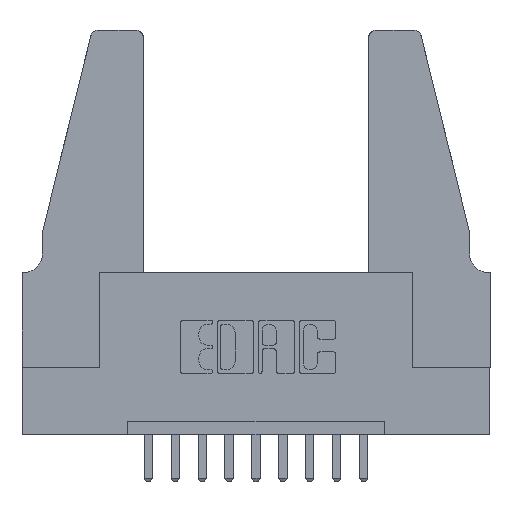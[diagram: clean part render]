
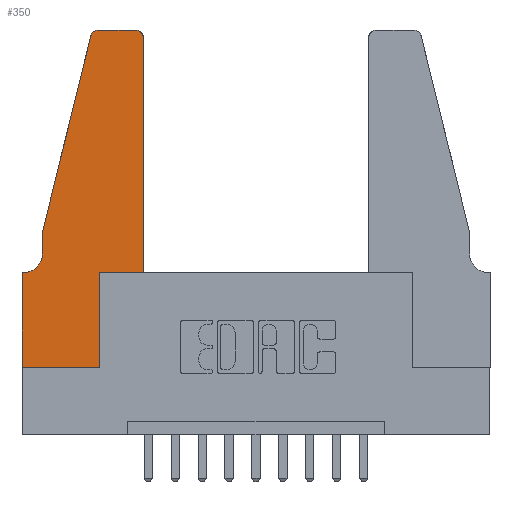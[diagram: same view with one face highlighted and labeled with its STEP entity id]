
A CAD part, top view. The second image highlights one B-rep face of the part: STEP entity #350.
In plain terms, the highlighted planar face has unit normal (0, 0, 1).
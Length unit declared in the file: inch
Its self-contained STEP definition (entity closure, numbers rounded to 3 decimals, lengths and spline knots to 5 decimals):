
#40 = EDGE_CURVE ( 'NONE', #12148, #10804, #7948, .T. ) ;
#112 = CARTESIAN_POINT ( 'NONE',  ( 0.2865, 0., 0.37 ) ) ;
#146 = DIRECTION ( 'NONE',  ( 0., 0., 1. ) ) ;
#165 = DIRECTION ( 'NONE',  ( 0., 0., 1. ) ) ;
#336 = LINE ( 'NONE', #9665, #4794 ) ;
#350 = ADVANCED_FACE ( 'NONE', ( #13003 ), #9407, .T. ) ;
#484 = VERTEX_POINT ( 'NONE', #9982 ) ;
#587 = CARTESIAN_POINT ( 'NONE',  ( 0.4505, 0.35, 0.37 ) ) ;
#904 = ORIENTED_EDGE ( 'NONE', *, *, #8625, .T. ) ;
#1178 = EDGE_CURVE ( 'NONE', #2941, #2637, #1564, .T. ) ;
#1369 = ORIENTED_EDGE ( 'NONE', *, *, #12515, .T. ) ;
#1439 = CARTESIAN_POINT ( 'NONE',  ( 0.0755, 0.5, 0.37 ) ) ;
#1564 = LINE ( 'NONE', #9667, #9541 ) ;
#1947 = CARTESIAN_POINT ( 'NONE',  ( 0.0755, 0.5, 0.37 ) ) ;
#2086 = LINE ( 'NONE', #9489, #12978 ) ;
#2240 = CARTESIAN_POINT ( 'NONE',  ( 0.0055, 0.42, 0.37 ) ) ;
#2256 = LINE ( 'NONE', #587, #9693 ) ;
#2637 = VERTEX_POINT ( 'NONE', #3068 ) ;
#2775 = DIRECTION ( 'NONE',  ( 1., 0., 0. ) ) ;
#2941 = VERTEX_POINT ( 'NONE', #12126 ) ;
#3068 = CARTESIAN_POINT ( 'NONE',  ( 0.4505, 1.22, 0.37 ) ) ;
#3259 = CARTESIAN_POINT ( 'NONE',  ( 0.0055, 0.35, 0.37 ) ) ;
#3442 = DIRECTION ( 'NONE',  ( -1., 0., 0. ) ) ;
#3523 = AXIS2_PLACEMENT_3D ( 'NONE', #9601, #165, #10624 ) ;
#3945 = ORIENTED_EDGE ( 'NONE', *, *, #1178, .T. ) ;
#4208 = CARTESIAN_POINT ( 'NONE',  ( 0.2605, 1.25, 0.37 ) ) ;
#4266 = VECTOR ( 'NONE', #6578, 39.37008 ) ;
#4300 = CARTESIAN_POINT ( 'NONE',  ( 0.284, 1.25, 0.37 ) ) ;
#4306 = EDGE_CURVE ( 'NONE', #10760, #12148, #11775, .T. ) ;
#4363 = VERTEX_POINT ( 'NONE', #8695 ) ;
#4393 = DIRECTION ( 'NONE',  ( 0., 0., -1. ) ) ;
#4583 = VECTOR ( 'NONE', #5790, 39.37008 ) ;
#4794 = VECTOR ( 'NONE', #3442, 39.37008 ) ;
#5053 = ORIENTED_EDGE ( 'NONE', *, *, #9400, .T. ) ;
#5328 = VERTEX_POINT ( 'NONE', #3259 ) ;
#5356 = VERTEX_POINT ( 'NONE', #4300 ) ;
#5540 = LINE ( 'NONE', #4208, #12079 ) ;
#5725 = CIRCLE ( 'NONE', #3523, 0.03 ) ;
#5748 = CARTESIAN_POINT ( 'NONE',  ( 0.2865, 0.35, 0.37 ) ) ;
#5778 = DIRECTION ( 'NONE',  ( 0., 0., 1. ) ) ;
#5790 = DIRECTION ( 'NONE',  ( 0., 1., 0. ) ) ;
#5828 = DIRECTION ( 'NONE',  ( 1., 0., 0. ) ) ;
#6429 = DIRECTION ( 'NONE',  ( 0., 1., 0. ) ) ;
#6578 = DIRECTION ( 'NONE',  ( -0.239, -0.971, 0. ) ) ;
#6589 = EDGE_CURVE ( 'NONE', #5328, #4363, #336, .T. ) ;
#6986 = ORIENTED_EDGE ( 'NONE', *, *, #8814, .T. ) ;
#7058 = EDGE_CURVE ( 'NONE', #13311, #10262, #9336, .T. ) ;
#7067 = CARTESIAN_POINT ( 'NONE',  ( 0.0755, 0.5, 0.37 ) ) ;
#7328 = DIRECTION ( 'NONE',  ( 1., 0., 0. ) ) ;
#7453 = DIRECTION ( 'NONE',  ( 0., -1., 0. ) ) ;
#7715 = CARTESIAN_POINT ( 'NONE',  ( 0.25487, 1.22718, 0.37 ) ) ;
#7799 = DIRECTION ( 'NONE',  ( 1., 0., 0. ) ) ;
#7948 = LINE ( 'NONE', #7067, #10395 ) ;
#8350 = VECTOR ( 'NONE', #7799, 39.37008 ) ;
#8625 = EDGE_CURVE ( 'NONE', #12604, #5356, #5540, .T. ) ;
#8695 = CARTESIAN_POINT ( 'NONE',  ( 0., 0.35, 0.37 ) ) ;
#8771 = CIRCLE ( 'NONE', #12287, 0.07 ) ;
#8814 = EDGE_CURVE ( 'NONE', #2637, #12604, #5725, .T. ) ;
#9336 = LINE ( 'NONE', #11967, #8350 ) ;
#9337 = ORIENTED_EDGE ( 'NONE', *, *, #40, .T. ) ;
#9400 = EDGE_CURVE ( 'NONE', #5356, #10760, #11571, .T. ) ;
#9401 = ORIENTED_EDGE ( 'NONE', *, *, #7058, .T. ) ;
#9407 = PLANE ( 'NONE',  #10644 ) ;
#9489 = CARTESIAN_POINT ( 'NONE',  ( 0., 0., 0.37 ) ) ;
#9541 = VECTOR ( 'NONE', #6429, 39.37008 ) ;
#9569 = DIRECTION ( 'NONE',  ( -1., 0., 0. ) ) ;
#9601 = CARTESIAN_POINT ( 'NONE',  ( 0.4205, 1.22, 0.37 ) ) ;
#9665 = CARTESIAN_POINT ( 'NONE',  ( 0.0755, 0.35, 0.37 ) ) ;
#9667 = CARTESIAN_POINT ( 'NONE',  ( 0.4505, 0.35, 0.37 ) ) ;
#9693 = VECTOR ( 'NONE', #5828, 39.37008 ) ;
#9746 = LINE ( 'NONE', #5748, #4583 ) ;
#9982 = CARTESIAN_POINT ( 'NONE',  ( 0.2865, 0.35, 0.37 ) ) ;
#9988 = CARTESIAN_POINT ( 'NONE',  ( 0.284, 1.22, 0.37 ) ) ;
#10087 = CARTESIAN_POINT ( 'NONE',  ( 0.4205, 1.25, 0.37 ) ) ;
#10262 = VERTEX_POINT ( 'NONE', #112 ) ;
#10395 = VECTOR ( 'NONE', #12257, 39.37008 ) ;
#10624 = DIRECTION ( 'NONE',  ( 1., 0., 0. ) ) ;
#10632 = EDGE_CURVE ( 'NONE', #4363, #13311, #2086, .T. ) ;
#10644 = AXIS2_PLACEMENT_3D ( 'NONE', #12687, #146, #7328 ) ;
#10760 = VERTEX_POINT ( 'NONE', #7715 ) ;
#10804 = VERTEX_POINT ( 'NONE', #13168 ) ;
#10815 = CARTESIAN_POINT ( 'NONE',  ( 0., 0., 0.37 ) ) ;
#10833 = AXIS2_PLACEMENT_3D ( 'NONE', #9988, #5778, #2775 ) ;
#10902 = EDGE_CURVE ( 'NONE', #484, #2941, #2256, .T. ) ;
#11190 = ORIENTED_EDGE ( 'NONE', *, *, #6589, .T. ) ;
#11514 = DIRECTION ( 'NONE',  ( -1., 0., 0. ) ) ;
#11571 = CIRCLE ( 'NONE', #10833, 0.03 ) ;
#11775 = LINE ( 'NONE', #1439, #4266 ) ;
#11967 = CARTESIAN_POINT ( 'NONE',  ( 0., 0., 0.37 ) ) ;
#12079 = VECTOR ( 'NONE', #11514, 39.37008 ) ;
#12126 = CARTESIAN_POINT ( 'NONE',  ( 0.4505, 0.35, 0.37 ) ) ;
#12148 = VERTEX_POINT ( 'NONE', #1947 ) ;
#12257 = DIRECTION ( 'NONE',  ( 0., -1., 0. ) ) ;
#12287 = AXIS2_PLACEMENT_3D ( 'NONE', #2240, #4393, #9569 ) ;
#12317 = ORIENTED_EDGE ( 'NONE', *, *, #4306, .T. ) ;
#12406 = ORIENTED_EDGE ( 'NONE', *, *, #10902, .T. ) ;
#12450 = ORIENTED_EDGE ( 'NONE', *, *, #13085, .T. ) ;
#12515 = EDGE_CURVE ( 'NONE', #10262, #484, #9746, .T. ) ;
#12604 = VERTEX_POINT ( 'NONE', #10087 ) ;
#12687 = CARTESIAN_POINT ( 'NONE',  ( 0., 0.35, 0.37 ) ) ;
#12978 = VECTOR ( 'NONE', #7453, 39.37008 ) ;
#13003 = FACE_OUTER_BOUND ( 'NONE', #13226, .T. ) ;
#13085 = EDGE_CURVE ( 'NONE', #10804, #5328, #8771, .T. ) ;
#13168 = CARTESIAN_POINT ( 'NONE',  ( 0.0755, 0.42, 0.37 ) ) ;
#13226 = EDGE_LOOP ( 'NONE', ( #904, #5053, #12317, #9337, #12450, #11190, #13303, #9401, #1369, #12406, #3945, #6986 ) ) ;
#13303 = ORIENTED_EDGE ( 'NONE', *, *, #10632, .T. ) ;
#13311 = VERTEX_POINT ( 'NONE', #10815 ) ;
